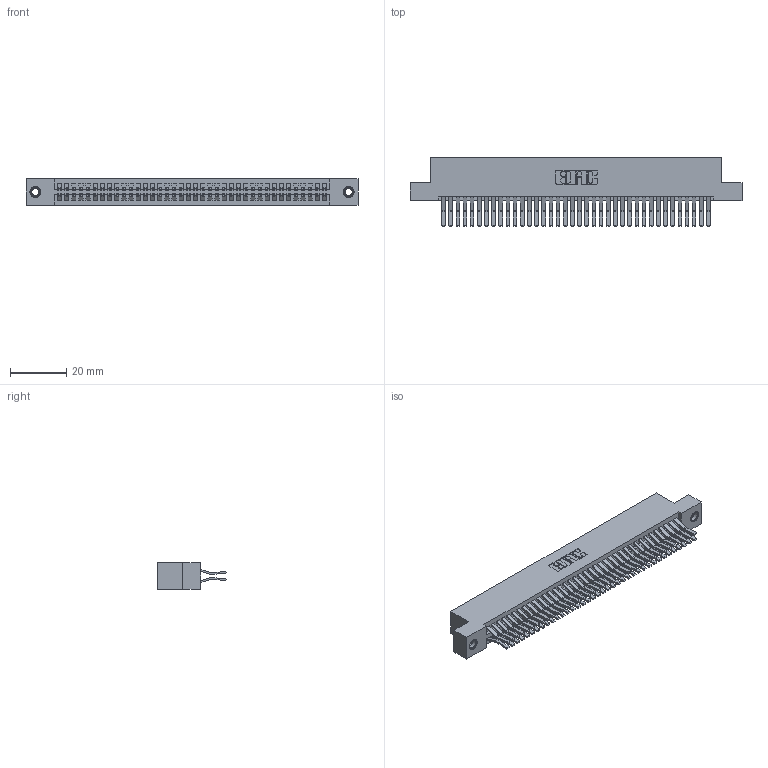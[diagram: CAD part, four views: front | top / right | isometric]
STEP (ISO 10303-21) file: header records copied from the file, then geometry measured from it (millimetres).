
FILE_DESCRIPTION (( 'STEP AP203' ), '1' );
FILE_NAME ('345-076-560-207.STEP', '2018-10-02T18:37:56', ( '' ), ( '' ), 'SwSTEP 2.0', 'SolidWorks 2016', '' );
FILE_SCHEMA (( 'CONFIG_CONTROL_DESIGN' ));
Length unit declared in the file: inch
Products named in the file (4): 345-076-560-207; 345 Part_Flush Mounting Lugs - 0.156 Dia-TI; 345-250-001_345-250-005-103; 345-292-001_560 Tail
Assembly tree (79 placements, depth 2):
  345-076-560-207
    345 Part_Flush Mounting Lugs - 0.156 Dia-TI
    345-292-001_560 Tail  x76
    345-250-001_345-250-005-103  x2
Bounding box: 117.73 x 24.45 x 9.4 mm (x, y, z)
Volume: 11883.8 mm3; surface area: 18797.9 mm2
Topology: 79 solids, 79 shells, 4138 faces, 12257 edges, 8062 vertices
Faces by surface type: plane 2620, cylinder 1502, cone 12, torus 4
Entity records: 31628 total; most frequent: CARTESIAN_POINT 5287, ORIENTED_EDGE 5214, DIRECTION 4697, EDGE_CURVE 2607, LINE 2299, VECTOR 2299, VERTEX_POINT 1732, AXIS2_PLACEMENT_3D 1199
